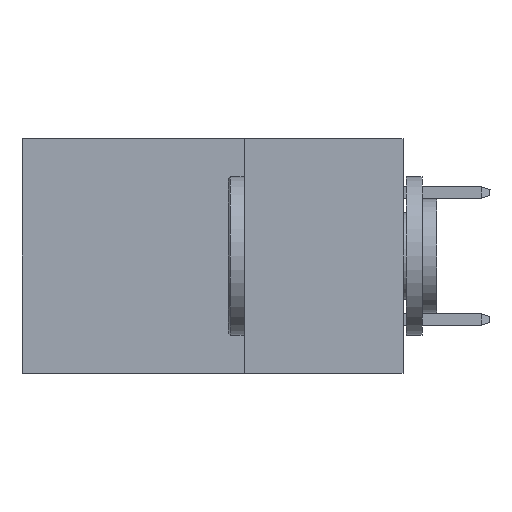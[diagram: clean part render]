
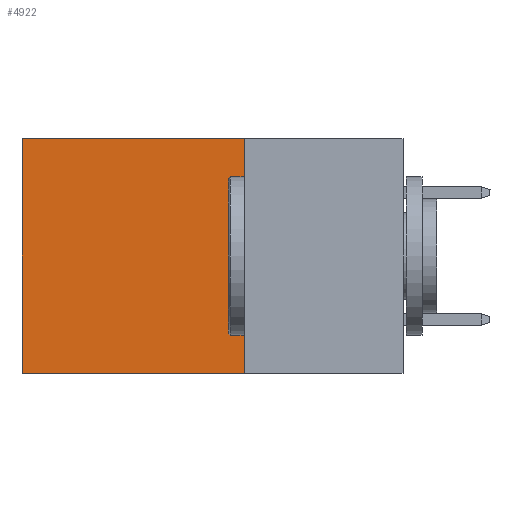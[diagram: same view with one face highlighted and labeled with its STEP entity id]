
A CAD part, left-side view. The second image highlights one B-rep face of the part: STEP entity #4922.
In plain terms, the highlighted planar face has unit normal (-1, 0, 0).
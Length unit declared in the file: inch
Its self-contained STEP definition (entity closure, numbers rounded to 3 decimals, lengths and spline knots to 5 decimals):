
#203 = EDGE_CURVE ( 'NONE', #7482, #9671, #5434, .T. ) ;
#220 = DIRECTION ( 'NONE',  ( 1., 0., 0. ) ) ;
#1124 = ORIENTED_EDGE ( 'NONE', *, *, #2151, .T. ) ;
#1147 = CARTESIAN_POINT ( 'NONE',  ( 0.2875, 0.25, 0. ) ) ;
#1643 = CARTESIAN_POINT ( 'NONE',  ( 0.2875, 0.6, 0. ) ) ;
#2151 = EDGE_CURVE ( 'NONE', #9671, #17206, #18561, .T. ) ;
#2972 = CARTESIAN_POINT ( 'NONE',  ( 0.2875, 0.25, 0. ) ) ;
#3975 = CARTESIAN_POINT ( 'NONE',  ( 0.2875, 0.25, 0. ) ) ;
#4189 = DIRECTION ( 'NONE',  ( 0., 0., -1. ) ) ;
#4922 = ADVANCED_FACE ( 'NONE', ( #13667 ), #11805, .F. ) ;
#5434 = LINE ( 'NONE', #3975, #13177 ) ;
#5568 = LINE ( 'NONE', #1147, #13038 ) ;
#6230 = EDGE_CURVE ( 'NONE', #11495, #17206, #12104, .T. ) ;
#6628 = VECTOR ( 'NONE', #11896, 39.37008 ) ;
#6986 = AXIS2_PLACEMENT_3D ( 'NONE', #2972, #220, #8969 ) ;
#7264 = ORIENTED_EDGE ( 'NONE', *, *, #203, .T. ) ;
#7482 = VERTEX_POINT ( 'NONE', #11258 ) ;
#8969 = DIRECTION ( 'NONE',  ( 0., 0., -1. ) ) ;
#9194 = CARTESIAN_POINT ( 'NONE',  ( 0.2875, 0.25, -0.37 ) ) ;
#9449 = CARTESIAN_POINT ( 'NONE',  ( 0.2875, 0.6, -0.37 ) ) ;
#9671 = VERTEX_POINT ( 'NONE', #1643 ) ;
#9959 = DIRECTION ( 'NONE',  ( 0., 1., 0. ) ) ;
#10112 = ORIENTED_EDGE ( 'NONE', *, *, #6230, .F. ) ;
#11258 = CARTESIAN_POINT ( 'NONE',  ( 0.2875, 0.25, 0. ) ) ;
#11495 = VERTEX_POINT ( 'NONE', #9194 ) ;
#11805 = PLANE ( 'NONE',  #6986 ) ;
#11896 = DIRECTION ( 'NONE',  ( 0., 1., 0. ) ) ;
#12104 = LINE ( 'NONE', #13670, #6628 ) ;
#13038 = VECTOR ( 'NONE', #4189, 39.37008 ) ;
#13177 = VECTOR ( 'NONE', #9959, 39.37008 ) ;
#13667 = FACE_OUTER_BOUND ( 'NONE', #15045, .T. ) ;
#13670 = CARTESIAN_POINT ( 'NONE',  ( 0.2875, 0.25, -0.37 ) ) ;
#13745 = CARTESIAN_POINT ( 'NONE',  ( 0.2875, 0.6, 0. ) ) ;
#14546 = EDGE_CURVE ( 'NONE', #7482, #11495, #5568, .T. ) ;
#15045 = EDGE_LOOP ( 'NONE', ( #1124, #10112, #18794, #7264 ) ) ;
#15700 = VECTOR ( 'NONE', #18380, 39.37008 ) ;
#17206 = VERTEX_POINT ( 'NONE', #9449 ) ;
#18380 = DIRECTION ( 'NONE',  ( 0., 0., -1. ) ) ;
#18561 = LINE ( 'NONE', #13745, #15700 ) ;
#18794 = ORIENTED_EDGE ( 'NONE', *, *, #14546, .F. ) ;
